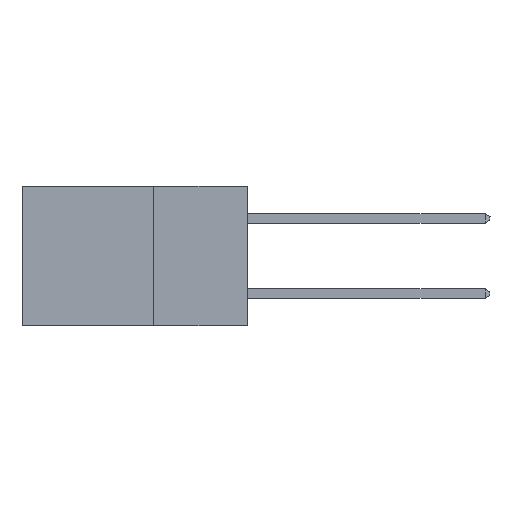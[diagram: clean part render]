
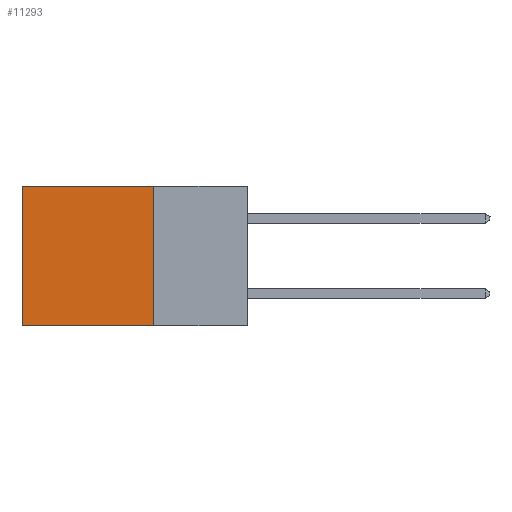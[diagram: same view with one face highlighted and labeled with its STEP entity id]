
A CAD part, left-side view. The second image highlights one B-rep face of the part: STEP entity #11293.
In plain terms, the highlighted planar face has unit normal (-1, 0, 0).
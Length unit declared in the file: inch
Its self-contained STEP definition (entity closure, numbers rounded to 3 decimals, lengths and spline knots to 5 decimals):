
#475 = AXIS2_PLACEMENT_3D ( 'NONE', #8631, #10410, #690 ) ;
#690 = DIRECTION ( 'NONE',  ( 0., 0., -1. ) ) ;
#743 = PLANE ( 'NONE',  #475 ) ;
#1425 = VECTOR ( 'NONE', #1542, 39.37008 ) ;
#1542 = DIRECTION ( 'NONE',  ( 0., 0., -1. ) ) ;
#2232 = VERTEX_POINT ( 'NONE', #3924 ) ;
#2305 = ORIENTED_EDGE ( 'NONE', *, *, #3794, .T. ) ;
#2495 = ORIENTED_EDGE ( 'NONE', *, *, #6250, .T. ) ;
#2823 = CARTESIAN_POINT ( 'NONE',  ( 0.2615, 0.25, 0. ) ) ;
#2846 = EDGE_CURVE ( 'NONE', #6000, #6388, #5197, .T. ) ;
#2876 = VECTOR ( 'NONE', #7223, 39.37008 ) ;
#3655 = DIRECTION ( 'NONE',  ( 0., 0., -1. ) ) ;
#3794 = EDGE_CURVE ( 'NONE', #6000, #10255, #9874, .T. ) ;
#3924 = CARTESIAN_POINT ( 'NONE',  ( 0.2615, 0.6, -0.37 ) ) ;
#4430 = CARTESIAN_POINT ( 'NONE',  ( 0.2615, 0.6, -0.37 ) ) ;
#4613 = CARTESIAN_POINT ( 'NONE',  ( 0.2615, 0.25, -0.37 ) ) ;
#5197 = LINE ( 'NONE', #8787, #6429 ) ;
#5495 = CARTESIAN_POINT ( 'NONE',  ( 0.2615, 0.6, 0. ) ) ;
#5982 = VECTOR ( 'NONE', #9020, 39.37008 ) ;
#6000 = VERTEX_POINT ( 'NONE', #2823 ) ;
#6121 = LINE ( 'NONE', #4430, #1425 ) ;
#6250 = EDGE_CURVE ( 'NONE', #10255, #2232, #6121, .T. ) ;
#6388 = VERTEX_POINT ( 'NONE', #6626 ) ;
#6429 = VECTOR ( 'NONE', #3655, 39.37008 ) ;
#6626 = CARTESIAN_POINT ( 'NONE',  ( 0.2615, 0.25, -0.37 ) ) ;
#7223 = DIRECTION ( 'NONE',  ( 0., 1., 0. ) ) ;
#8137 = CARTESIAN_POINT ( 'NONE',  ( 0.2615, 0.25, 0. ) ) ;
#8631 = CARTESIAN_POINT ( 'NONE',  ( 0.2615, 0.25, -0.37 ) ) ;
#8787 = CARTESIAN_POINT ( 'NONE',  ( 0.2615, 0.25, -0.37 ) ) ;
#8832 = EDGE_CURVE ( 'NONE', #6388, #2232, #9191, .T. ) ;
#9020 = DIRECTION ( 'NONE',  ( 0., 1., 0. ) ) ;
#9191 = LINE ( 'NONE', #4613, #5982 ) ;
#9874 = LINE ( 'NONE', #8137, #2876 ) ;
#10106 = ORIENTED_EDGE ( 'NONE', *, *, #8832, .F. ) ;
#10255 = VERTEX_POINT ( 'NONE', #5495 ) ;
#10369 = EDGE_LOOP ( 'NONE', ( #2495, #10106, #10877, #2305 ) ) ;
#10410 = DIRECTION ( 'NONE',  ( 1., 0., 0. ) ) ;
#10877 = ORIENTED_EDGE ( 'NONE', *, *, #2846, .F. ) ;
#11293 = ADVANCED_FACE ( 'NONE', ( #11531 ), #743, .F. ) ;
#11531 = FACE_OUTER_BOUND ( 'NONE', #10369, .T. ) ;
